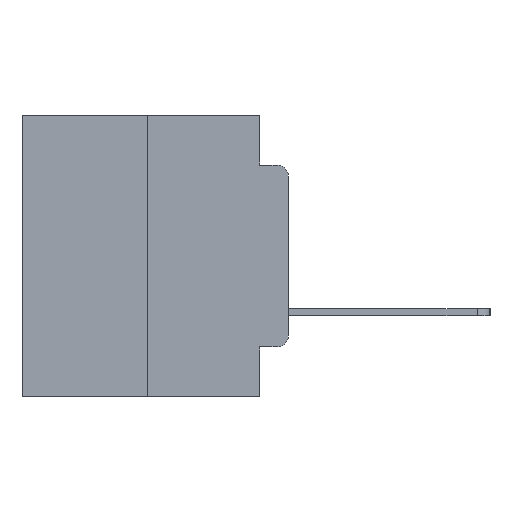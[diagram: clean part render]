
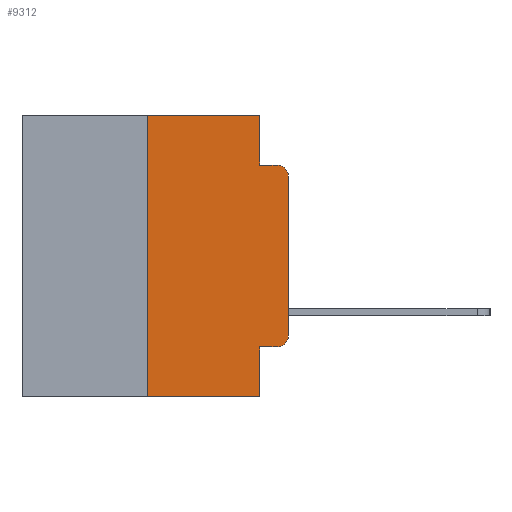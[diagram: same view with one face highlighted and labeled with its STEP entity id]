
A CAD part, left-side view. The second image highlights one B-rep face of the part: STEP entity #9312.
In plain terms, the highlighted planar face has unit normal (-1, 0, 0).
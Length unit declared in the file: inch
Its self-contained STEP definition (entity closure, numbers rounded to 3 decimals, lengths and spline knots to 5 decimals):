
#672 = CARTESIAN_POINT ( 'NONE',  ( 0., 0.051, 0. ) ) ;
#682 = CARTESIAN_POINT ( 'NONE',  ( 0., 0.02, -0.0885 ) ) ;
#700 = CIRCLE ( 'NONE', #16811, 0.02 ) ;
#717 = CARTESIAN_POINT ( 'NONE',  ( 0., 0.473, 0. ) ) ;
#1853 = DIRECTION ( 'NONE',  ( 0., 0., -1. ) ) ;
#1979 = DIRECTION ( 'NONE',  ( 0., 0., -1. ) ) ;
#2356 = CARTESIAN_POINT ( 'NONE',  ( 0., 0.051, -0.0885 ) ) ;
#2622 = CARTESIAN_POINT ( 'NONE',  ( 0., 0.473, 0. ) ) ;
#2692 = ORIENTED_EDGE ( 'NONE', *, *, #5579, .T. ) ;
#2778 = LINE ( 'NONE', #7946, #19043 ) ;
#2852 = CARTESIAN_POINT ( 'NONE',  ( 0., 0.051, 0. ) ) ;
#3100 = EDGE_CURVE ( 'NONE', #25317, #16406, #15709, .T. ) ;
#3439 = VERTEX_POINT ( 'NONE', #12126 ) ;
#4001 = ORIENTED_EDGE ( 'NONE', *, *, #4347, .F. ) ;
#4131 = EDGE_CURVE ( 'NONE', #15676, #19445, #25806, .T. ) ;
#4330 = CARTESIAN_POINT ( 'NONE',  ( 0., 0.02, -0.3915 ) ) ;
#4347 = EDGE_CURVE ( 'NONE', #12103, #24237, #21250, .T. ) ;
#4670 = ORIENTED_EDGE ( 'NONE', *, *, #23148, .F. ) ;
#5579 = EDGE_CURVE ( 'NONE', #14081, #15676, #7425, .T. ) ;
#6468 = DIRECTION ( 'NONE',  ( 0., 0., -1. ) ) ;
#6958 = DIRECTION ( 'NONE',  ( 0., -1., 0. ) ) ;
#7425 = LINE ( 'NONE', #16005, #22995 ) ;
#7540 = FACE_OUTER_BOUND ( 'NONE', #11358, .T. ) ;
#7543 = LINE ( 'NONE', #2852, #18833 ) ;
#7946 = CARTESIAN_POINT ( 'NONE',  ( 0., 0.25, 0. ) ) ;
#8951 = PLANE ( 'NONE',  #21468 ) ;
#9203 = DIRECTION ( 'NONE',  ( 0., -1., 0. ) ) ;
#9312 = ADVANCED_FACE ( 'NONE', ( #7540 ), #8951, .F. ) ;
#10104 = DIRECTION ( 'NONE',  ( 0., 0., 1. ) ) ;
#10430 = CARTESIAN_POINT ( 'NONE',  ( 0., 0.051, -0.4115 ) ) ;
#11358 = EDGE_LOOP ( 'NONE', ( #2692, #14036, #25180, #25820, #4001, #4670, #16009, #22291, #17324, #23572 ) ) ;
#11369 = LINE ( 'NONE', #27243, #27413 ) ;
#11461 = CARTESIAN_POINT ( 'NONE',  ( 0., 0., -0.1085 ) ) ;
#11790 = CARTESIAN_POINT ( 'NONE',  ( 0., 0.051, -0.5 ) ) ;
#12103 = VERTEX_POINT ( 'NONE', #19399 ) ;
#12126 = CARTESIAN_POINT ( 'NONE',  ( 0., 0.02, -0.4115 ) ) ;
#12381 = AXIS2_PLACEMENT_3D ( 'NONE', #27128, #14594, #1853 ) ;
#13326 = DIRECTION ( 'NONE',  ( 0., 0., -1. ) ) ;
#14036 = ORIENTED_EDGE ( 'NONE', *, *, #4131, .T. ) ;
#14081 = VERTEX_POINT ( 'NONE', #19360 ) ;
#14278 = VECTOR ( 'NONE', #15103, 39.37008 ) ;
#14594 = DIRECTION ( 'NONE',  ( -1., 0., 0. ) ) ;
#14927 = LINE ( 'NONE', #2356, #14278 ) ;
#15103 = DIRECTION ( 'NONE',  ( 0., -1., 0. ) ) ;
#15289 = VECTOR ( 'NONE', #6958, 39.37008 ) ;
#15676 = VERTEX_POINT ( 'NONE', #11461 ) ;
#15709 = LINE ( 'NONE', #17328, #18677 ) ;
#16005 = CARTESIAN_POINT ( 'NONE',  ( 0., 0., 0. ) ) ;
#16009 = ORIENTED_EDGE ( 'NONE', *, *, #3100, .T. ) ;
#16096 = EDGE_CURVE ( 'NONE', #3439, #14081, #700, .T. ) ;
#16406 = VERTEX_POINT ( 'NONE', #11790 ) ;
#16811 = AXIS2_PLACEMENT_3D ( 'NONE', #4330, #19183, #6468 ) ;
#17324 = ORIENTED_EDGE ( 'NONE', *, *, #17515, .T. ) ;
#17328 = CARTESIAN_POINT ( 'NONE',  ( 0., 0.473, -0.5 ) ) ;
#17515 = EDGE_CURVE ( 'NONE', #22062, #3439, #20893, .T. ) ;
#17572 = CARTESIAN_POINT ( 'NONE',  ( 0., 0.051, -0.4115 ) ) ;
#18128 = DIRECTION ( 'NONE',  ( 0., 0., 1. ) ) ;
#18677 = VECTOR ( 'NONE', #23577, 39.37008 ) ;
#18833 = VECTOR ( 'NONE', #19731, 39.37008 ) ;
#18915 = EDGE_CURVE ( 'NONE', #22062, #16406, #7543, .T. ) ;
#19043 = VECTOR ( 'NONE', #10104, 39.37008 ) ;
#19183 = DIRECTION ( 'NONE',  ( -1., 0., 0. ) ) ;
#19360 = CARTESIAN_POINT ( 'NONE',  ( 0., 0., -0.3915 ) ) ;
#19399 = CARTESIAN_POINT ( 'NONE',  ( 0., 0.25, 0. ) ) ;
#19445 = VERTEX_POINT ( 'NONE', #682 ) ;
#19731 = DIRECTION ( 'NONE',  ( 0., 0., -1. ) ) ;
#20893 = LINE ( 'NONE', #17572, #15289 ) ;
#21250 = LINE ( 'NONE', #717, #26120 ) ;
#21468 = AXIS2_PLACEMENT_3D ( 'NONE', #2622, #25884, #13326 ) ;
#22062 = VERTEX_POINT ( 'NONE', #10430 ) ;
#22291 = ORIENTED_EDGE ( 'NONE', *, *, #18915, .F. ) ;
#22486 = CARTESIAN_POINT ( 'NONE',  ( 0., 0.051, -0.0885 ) ) ;
#22995 = VECTOR ( 'NONE', #18128, 39.37008 ) ;
#23148 = EDGE_CURVE ( 'NONE', #25317, #12103, #2778, .T. ) ;
#23572 = ORIENTED_EDGE ( 'NONE', *, *, #16096, .T. ) ;
#23577 = DIRECTION ( 'NONE',  ( 0., -1., 0. ) ) ;
#23603 = CARTESIAN_POINT ( 'NONE',  ( 0., 0.25, -0.5 ) ) ;
#24237 = VERTEX_POINT ( 'NONE', #672 ) ;
#24551 = EDGE_CURVE ( 'NONE', #24237, #27234, #11369, .T. ) ;
#25180 = ORIENTED_EDGE ( 'NONE', *, *, #25911, .F. ) ;
#25317 = VERTEX_POINT ( 'NONE', #23603 ) ;
#25806 = CIRCLE ( 'NONE', #12381, 0.02 ) ;
#25820 = ORIENTED_EDGE ( 'NONE', *, *, #24551, .F. ) ;
#25884 = DIRECTION ( 'NONE',  ( 1., 0., 0. ) ) ;
#25911 = EDGE_CURVE ( 'NONE', #27234, #19445, #14927, .T. ) ;
#26120 = VECTOR ( 'NONE', #9203, 39.37008 ) ;
#27128 = CARTESIAN_POINT ( 'NONE',  ( 0., 0.02, -0.1085 ) ) ;
#27234 = VERTEX_POINT ( 'NONE', #22486 ) ;
#27243 = CARTESIAN_POINT ( 'NONE',  ( 0., 0.051, 0. ) ) ;
#27413 = VECTOR ( 'NONE', #1979, 39.37008 ) ;
